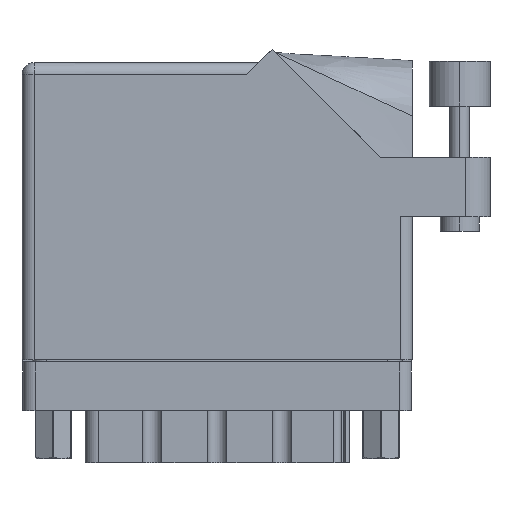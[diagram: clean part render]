
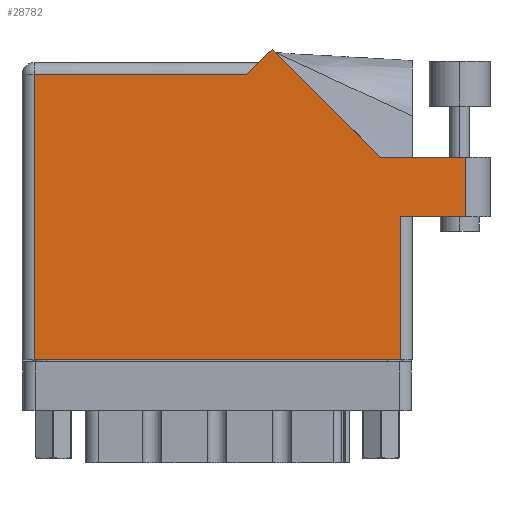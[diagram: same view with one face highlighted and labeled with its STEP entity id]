
A CAD part, front view. The second image highlights one B-rep face of the part: STEP entity #28782.
In plain terms, the highlighted face is planar.
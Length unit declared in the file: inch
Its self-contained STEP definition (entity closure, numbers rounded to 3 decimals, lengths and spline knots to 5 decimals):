
#196 = CARTESIAN_POINT ( 'NONE',  ( 0., 1.468, 0. ) ) ;
#1395 = CARTESIAN_POINT ( 'NONE',  ( 1.28771, 1.60071, 0. ) ) ;
#1525 = EDGE_CURVE ( 'NONE', #19953, #16495, #35930, .T. ) ;
#1561 = LINE ( 'NONE', #25506, #10596 ) ;
#1864 = CARTESIAN_POINT ( 'NONE',  ( 2.285, 1.044, 0. ) ) ;
#1941 = CARTESIAN_POINT ( 'NONE',  ( 0., 1.53, 0. ) ) ;
#2363 = CARTESIAN_POINT ( 'NONE',  ( 2.41, 1.044, 0. ) ) ;
#2397 = ORIENTED_EDGE ( 'NONE', *, *, #19040, .T. ) ;
#2434 = CARTESIAN_POINT ( 'NONE',  ( 0.062, 0., 0. ) ) ;
#2616 = DIRECTION ( 'NONE',  ( 0., -1., 0. ) ) ;
#2698 = VECTOR ( 'NONE', #2616, 39.37008 ) ;
#3049 = VERTEX_POINT ( 'NONE', #18183 ) ;
#3421 = DIRECTION ( 'NONE',  ( -0.707, -0.707, 0. ) ) ;
#4006 = VECTOR ( 'NONE', #26172, 39.37008 ) ;
#4676 = ORIENTED_EDGE ( 'NONE', *, *, #36578, .T. ) ;
#4812 = VECTOR ( 'NONE', #25309, 39.37008 ) ;
#5810 = DIRECTION ( 'NONE',  ( -1., 0., 0. ) ) ;
#5955 = VECTOR ( 'NONE', #23794, 39.37008 ) ;
#6954 = LINE ( 'NONE', #8993, #30507 ) ;
#8993 = CARTESIAN_POINT ( 'NONE',  ( 2.01, 0.737, 0. ) ) ;
#9739 = EDGE_CURVE ( 'NONE', #30544, #19953, #35493, .T. ) ;
#9787 = CARTESIAN_POINT ( 'NONE',  ( 2.285, 0.737, 0. ) ) ;
#10300 = VERTEX_POINT ( 'NONE', #31956 ) ;
#10596 = VECTOR ( 'NONE', #40761, 39.37008 ) ;
#12191 = EDGE_CURVE ( 'NONE', #16495, #23550, #6954, .T. ) ;
#13769 = DIRECTION ( 'NONE',  ( 0., 0., -1. ) ) ;
#14433 = LINE ( 'NONE', #2363, #18088 ) ;
#16495 = VERTEX_POINT ( 'NONE', #30101 ) ;
#17318 = PLANE ( 'NONE',  #25701 ) ;
#18088 = VECTOR ( 'NONE', #36860, 39.37008 ) ;
#18183 = CARTESIAN_POINT ( 'NONE',  ( 1.84442, 1.044, 0. ) ) ;
#18987 = DIRECTION ( 'NONE',  ( -1., 0., 0. ) ) ;
#19040 = EDGE_CURVE ( 'NONE', #44819, #3049, #14433, .T. ) ;
#19131 = CARTESIAN_POINT ( 'NONE',  ( 1.217, 1.53, 0. ) ) ;
#19953 = VERTEX_POINT ( 'NONE', #31784 ) ;
#20018 = DIRECTION ( 'NONE',  ( 1., 0., 0. ) ) ;
#22175 = ORIENTED_EDGE ( 'NONE', *, *, #9739, .T. ) ;
#22378 = EDGE_LOOP ( 'NONE', ( #36162, #32564, #2397, #31417, #35729, #4676, #42856, #22175, #43430 ) ) ;
#23550 = VERTEX_POINT ( 'NONE', #9787 ) ;
#23794 = DIRECTION ( 'NONE',  ( 1., 0., 0. ) ) ;
#24665 = LINE ( 'NONE', #19131, #42656 ) ;
#25309 = DIRECTION ( 'NONE',  ( -0.707, 0.707, 0. ) ) ;
#25506 = CARTESIAN_POINT ( 'NONE',  ( 2.285, 1.044, 0. ) ) ;
#25701 = AXIS2_PLACEMENT_3D ( 'NONE', #1941, #13769, #5810 ) ;
#26172 = DIRECTION ( 'NONE',  ( 0., 1., 0. ) ) ;
#26213 = CARTESIAN_POINT ( 'NONE',  ( 0.062, 1.468, 0. ) ) ;
#28782 = ADVANCED_FACE ( 'NONE', ( #32585 ), #17318, .F. ) ;
#28845 = CARTESIAN_POINT ( 'NONE',  ( 1.84442, 1.044, 0. ) ) ;
#29463 = EDGE_CURVE ( 'NONE', #23550, #44819, #1561, .T. ) ;
#30101 = CARTESIAN_POINT ( 'NONE',  ( 1.948, 0.737, 0. ) ) ;
#30507 = VECTOR ( 'NONE', #20018, 39.37008 ) ;
#30544 = VERTEX_POINT ( 'NONE', #38919 ) ;
#30888 = EDGE_CURVE ( 'NONE', #3049, #31601, #31368, .T. ) ;
#31368 = LINE ( 'NONE', #28845, #4812 ) ;
#31417 = ORIENTED_EDGE ( 'NONE', *, *, #30888, .T. ) ;
#31601 = VERTEX_POINT ( 'NONE', #1395 ) ;
#31784 = CARTESIAN_POINT ( 'NONE',  ( 1.948, 0., 0. ) ) ;
#31834 = EDGE_CURVE ( 'NONE', #31601, #10300, #24665, .T. ) ;
#31956 = CARTESIAN_POINT ( 'NONE',  ( 1.155, 1.468, 0. ) ) ;
#32564 = ORIENTED_EDGE ( 'NONE', *, *, #29463, .T. ) ;
#32585 = FACE_OUTER_BOUND ( 'NONE', #22378, .T. ) ;
#35493 = LINE ( 'NONE', #38389, #5955 ) ;
#35729 = ORIENTED_EDGE ( 'NONE', *, *, #31834, .T. ) ;
#35930 = LINE ( 'NONE', #40291, #4006 ) ;
#36162 = ORIENTED_EDGE ( 'NONE', *, *, #12191, .T. ) ;
#36578 = EDGE_CURVE ( 'NONE', #10300, #46227, #42302, .T. ) ;
#36860 = DIRECTION ( 'NONE',  ( -1., 0., 0. ) ) ;
#38095 = VECTOR ( 'NONE', #18987, 39.37008 ) ;
#38389 = CARTESIAN_POINT ( 'NONE',  ( 0., 0., 0. ) ) ;
#38919 = CARTESIAN_POINT ( 'NONE',  ( 0.062, 0., 0. ) ) ;
#40291 = CARTESIAN_POINT ( 'NONE',  ( 1.948, 0.737, 0. ) ) ;
#40665 = LINE ( 'NONE', #2434, #2698 ) ;
#40761 = DIRECTION ( 'NONE',  ( 0., 1., 0. ) ) ;
#42302 = LINE ( 'NONE', #196, #38095 ) ;
#42656 = VECTOR ( 'NONE', #3421, 39.37008 ) ;
#42856 = ORIENTED_EDGE ( 'NONE', *, *, #48073, .T. ) ;
#43430 = ORIENTED_EDGE ( 'NONE', *, *, #1525, .T. ) ;
#44819 = VERTEX_POINT ( 'NONE', #1864 ) ;
#46227 = VERTEX_POINT ( 'NONE', #26213 ) ;
#48073 = EDGE_CURVE ( 'NONE', #46227, #30544, #40665, .T. ) ;
